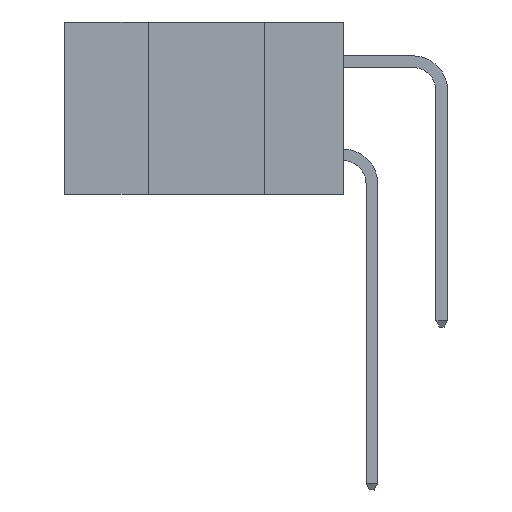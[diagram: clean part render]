
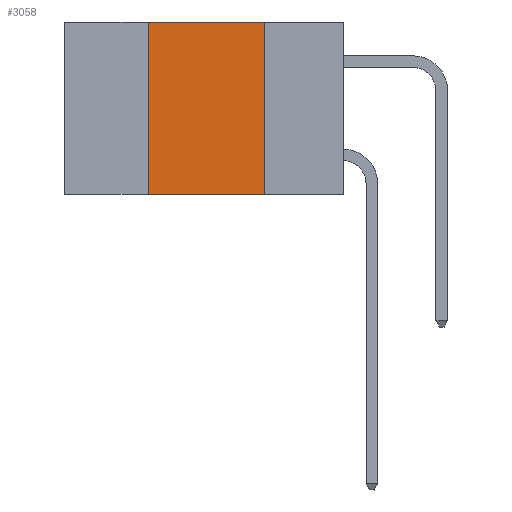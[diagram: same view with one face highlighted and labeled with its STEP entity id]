
A CAD part, left-side view. The second image highlights one B-rep face of the part: STEP entity #3058.
In plain terms, the highlighted planar face has unit normal (-1, 0, 0).
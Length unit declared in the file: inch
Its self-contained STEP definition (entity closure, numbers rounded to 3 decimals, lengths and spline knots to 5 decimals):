
#240 = EDGE_CURVE ( 'NONE', #2387, #7855, #20345, .T. ) ;
#1379 = ORIENTED_EDGE ( 'NONE', *, *, #3037, .F. ) ;
#1386 = LINE ( 'NONE', #11920, #11074 ) ;
#1526 = VECTOR ( 'NONE', #18163, 39.37008 ) ;
#1562 = EDGE_CURVE ( 'NONE', #2387, #3078, #1386, .T. ) ;
#2387 = VERTEX_POINT ( 'NONE', #4806 ) ;
#3037 = EDGE_CURVE ( 'NONE', #7855, #4644, #12389, .T. ) ;
#3058 = ADVANCED_FACE ( 'NONE', ( #20749 ), #12508, .F. ) ;
#3078 = VERTEX_POINT ( 'NONE', #21907 ) ;
#4644 = VERTEX_POINT ( 'NONE', #15685 ) ;
#4806 = CARTESIAN_POINT ( 'NONE',  ( 0., 0.42, -0.37 ) ) ;
#5808 = CARTESIAN_POINT ( 'NONE',  ( 0., 0.6, 0. ) ) ;
#6589 = ORIENTED_EDGE ( 'NONE', *, *, #240, .F. ) ;
#7210 = ORIENTED_EDGE ( 'NONE', *, *, #1562, .T. ) ;
#7855 = VERTEX_POINT ( 'NONE', #9738 ) ;
#8734 = LINE ( 'NONE', #21212, #17654 ) ;
#9738 = CARTESIAN_POINT ( 'NONE',  ( 0., 0.42, 0. ) ) ;
#11068 = ORIENTED_EDGE ( 'NONE', *, *, #17503, .F. ) ;
#11074 = VECTOR ( 'NONE', #12629, 39.37008 ) ;
#11682 = EDGE_LOOP ( 'NONE', ( #11068, #1379, #6589, #7210 ) ) ;
#11920 = CARTESIAN_POINT ( 'NONE',  ( 0., 0.6, -0.37 ) ) ;
#12389 = LINE ( 'NONE', #5808, #1526 ) ;
#12508 = PLANE ( 'NONE',  #24033 ) ;
#12629 = DIRECTION ( 'NONE',  ( 0., -1., 0. ) ) ;
#12665 = DIRECTION ( 'NONE',  ( 0., 0., 1. ) ) ;
#12805 = CARTESIAN_POINT ( 'NONE',  ( 0., 0.42, 0. ) ) ;
#12947 = CARTESIAN_POINT ( 'NONE',  ( 0., 0.6, 0. ) ) ;
#15276 = VECTOR ( 'NONE', #12665, 39.37008 ) ;
#15685 = CARTESIAN_POINT ( 'NONE',  ( 0., 0.17, 0. ) ) ;
#17503 = EDGE_CURVE ( 'NONE', #4644, #3078, #8734, .T. ) ;
#17654 = VECTOR ( 'NONE', #19404, 39.37008 ) ;
#18163 = DIRECTION ( 'NONE',  ( 0., -1., 0. ) ) ;
#19404 = DIRECTION ( 'NONE',  ( 0., 0., -1. ) ) ;
#20345 = LINE ( 'NONE', #12805, #15276 ) ;
#20749 = FACE_OUTER_BOUND ( 'NONE', #11682, .T. ) ;
#21212 = CARTESIAN_POINT ( 'NONE',  ( 0., 0.17, 0. ) ) ;
#21907 = CARTESIAN_POINT ( 'NONE',  ( 0., 0.17, -0.37 ) ) ;
#22539 = DIRECTION ( 'NONE',  ( 0., 0., -1. ) ) ;
#22598 = DIRECTION ( 'NONE',  ( 1., 0., 0. ) ) ;
#24033 = AXIS2_PLACEMENT_3D ( 'NONE', #12947, #22598, #22539 ) ;
